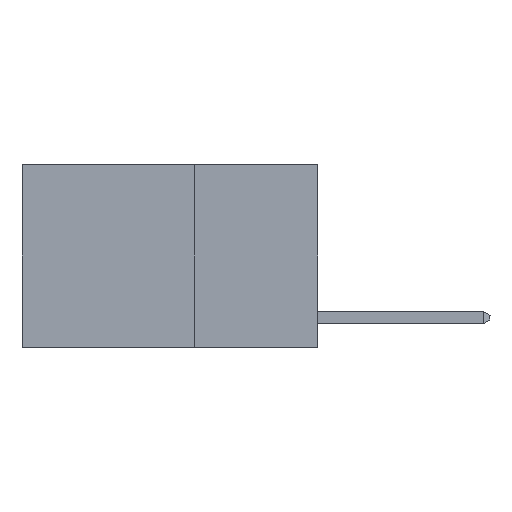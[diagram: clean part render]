
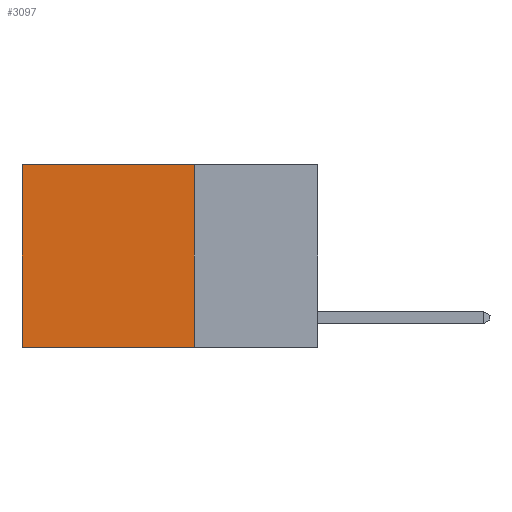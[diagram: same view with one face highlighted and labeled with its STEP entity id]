
A CAD part, left-side view. The second image highlights one B-rep face of the part: STEP entity #3097.
In plain terms, the highlighted planar face has unit normal (-1, 0, 0).
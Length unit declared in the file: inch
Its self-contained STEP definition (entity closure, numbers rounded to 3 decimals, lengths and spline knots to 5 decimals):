
#136 = EDGE_CURVE ( 'NONE', #8002, #144, #7312, .T. ) ;
#144 = VERTEX_POINT ( 'NONE', #2859 ) ;
#205 = CARTESIAN_POINT ( 'NONE',  ( 0.2625, 0.25, 0. ) ) ;
#287 = PLANE ( 'NONE',  #2728 ) ;
#569 = VECTOR ( 'NONE', #12509, 39.37008 ) ;
#751 = VERTEX_POINT ( 'NONE', #9311 ) ;
#774 = VERTEX_POINT ( 'NONE', #4197 ) ;
#922 = EDGE_LOOP ( 'NONE', ( #9376, #9439, #9476, #9504 ) ) ;
#1600 = VECTOR ( 'NONE', #12240, 39.37008 ) ;
#1897 = LINE ( 'NONE', #9272, #12168 ) ;
#2408 = CARTESIAN_POINT ( 'NONE',  ( 0.2625, 0.25, 0. ) ) ;
#2565 = EDGE_CURVE ( 'NONE', #751, #774, #8671, .T. ) ;
#2728 = AXIS2_PLACEMENT_3D ( 'NONE', #2408, #9481, #3444 ) ;
#2859 = CARTESIAN_POINT ( 'NONE',  ( 0.2625, 0.25, -0.37 ) ) ;
#3097 = ADVANCED_FACE ( 'NONE', ( #5911 ), #287, .F. ) ;
#3354 = DIRECTION ( 'NONE',  ( 0., 1., 0. ) ) ;
#3444 = DIRECTION ( 'NONE',  ( 0., 0., -1. ) ) ;
#3678 = EDGE_CURVE ( 'NONE', #8002, #751, #1897, .T. ) ;
#4197 = CARTESIAN_POINT ( 'NONE',  ( 0.2625, 0.6, -0.37 ) ) ;
#5359 = DIRECTION ( 'NONE',  ( 0., 1., 0. ) ) ;
#5734 = CARTESIAN_POINT ( 'NONE',  ( 0.2625, 0.25, 0. ) ) ;
#5743 = CARTESIAN_POINT ( 'NONE',  ( 0.2625, 0.6, 0. ) ) ;
#5911 = FACE_OUTER_BOUND ( 'NONE', #922, .T. ) ;
#7312 = LINE ( 'NONE', #5734, #1600 ) ;
#8002 = VERTEX_POINT ( 'NONE', #205 ) ;
#8016 = LINE ( 'NONE', #9470, #12859 ) ;
#8671 = LINE ( 'NONE', #5743, #569 ) ;
#9272 = CARTESIAN_POINT ( 'NONE',  ( 0.2625, 0.25, 0. ) ) ;
#9311 = CARTESIAN_POINT ( 'NONE',  ( 0.2625, 0.6, 0. ) ) ;
#9376 = ORIENTED_EDGE ( 'NONE', *, *, #2565, .T. ) ;
#9439 = ORIENTED_EDGE ( 'NONE', *, *, #10698, .F. ) ;
#9470 = CARTESIAN_POINT ( 'NONE',  ( 0.2625, 0.25, -0.37 ) ) ;
#9476 = ORIENTED_EDGE ( 'NONE', *, *, #136, .F. ) ;
#9481 = DIRECTION ( 'NONE',  ( 1., 0., 0. ) ) ;
#9504 = ORIENTED_EDGE ( 'NONE', *, *, #3678, .T. ) ;
#10698 = EDGE_CURVE ( 'NONE', #144, #774, #8016, .T. ) ;
#12168 = VECTOR ( 'NONE', #5359, 39.37008 ) ;
#12240 = DIRECTION ( 'NONE',  ( 0., 0., -1. ) ) ;
#12509 = DIRECTION ( 'NONE',  ( 0., 0., -1. ) ) ;
#12859 = VECTOR ( 'NONE', #3354, 39.37008 ) ;
